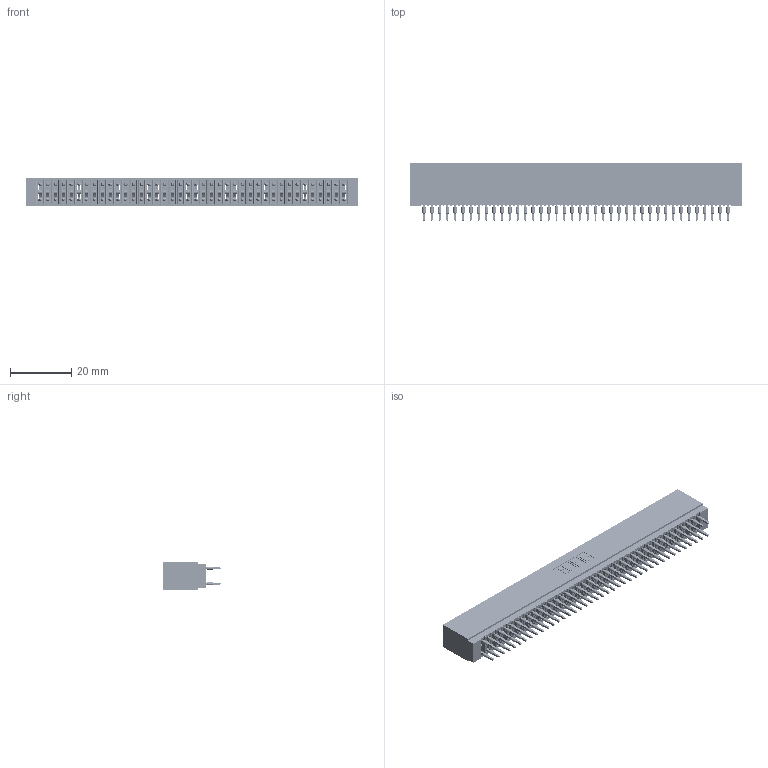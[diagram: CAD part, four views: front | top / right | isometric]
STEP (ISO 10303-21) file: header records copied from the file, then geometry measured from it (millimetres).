
FILE_DESCRIPTION (( 'STEP AP203' ), '1' );
FILE_NAME ('725-080-560-201.STEP', '2026-02-24T19:03:59', ( '' ), ( '' ), 'SwSTEP 2.0', 'SolidWorks 2023', '' );
FILE_SCHEMA (( 'CONFIG_CONTROL_DESIGN' ));
Length unit declared in the file: millimetre
Products named in the file (3): 745-292-001_560; 725 Part_Insulator Option - 01; 725-080-560-201
Assembly tree (81 placements, depth 2):
  725-080-560-201
    725 Part_Insulator Option - 01
    745-292-001_560  x80
Bounding box: 108.2 x 18.8 x 8.89 mm (x, y, z)
Volume: 8886.3 mm3; surface area: 19987.6 mm2
Topology: 81 solids, 81 shells, 7975 faces, 21814 edges, 13848 vertices
Faces by surface type: plane 4135, cylinder 1760, bspline 1600, torus 480
Entity records: 67901 total; most frequent: CARTESIAN_POINT 12281, ORIENTED_EDGE 11712, DIRECTION 10240, EDGE_CURVE 5856, VECTOR 5426, LINE 5426, VERTEX_POINT 3736, AXIS2_PLACEMENT_3D 2407
